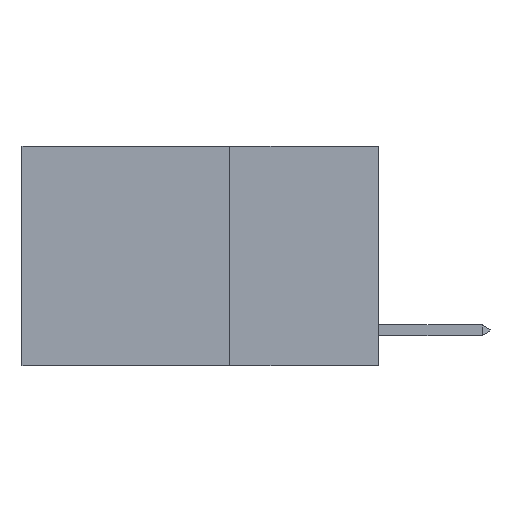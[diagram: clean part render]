
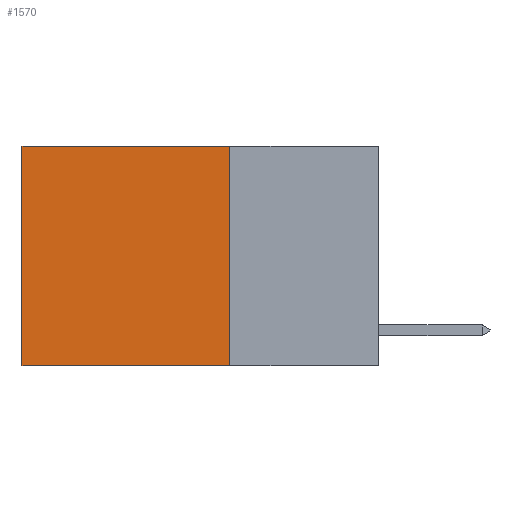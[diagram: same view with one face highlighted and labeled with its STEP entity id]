
A CAD part, left-side view. The second image highlights one B-rep face of the part: STEP entity #1570.
In plain terms, the highlighted planar face has unit normal (-1, 0, 0).
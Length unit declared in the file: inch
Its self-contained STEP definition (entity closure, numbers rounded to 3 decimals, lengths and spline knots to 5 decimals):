
#242 = ORIENTED_EDGE ( 'NONE', *, *, #7234, .T. ) ;
#733 = ORIENTED_EDGE ( 'NONE', *, *, #9183, .F. ) ;
#904 = ORIENTED_EDGE ( 'NONE', *, *, #3686, .T. ) ;
#1250 = VECTOR ( 'NONE', #5497, 39.37008 ) ;
#1519 = VERTEX_POINT ( 'NONE', #7907 ) ;
#1570 = ADVANCED_FACE ( 'NONE', ( #4399 ), #10146, .F. ) ;
#1814 = ORIENTED_EDGE ( 'NONE', *, *, #3489, .F. ) ;
#2199 = CARTESIAN_POINT ( 'NONE',  ( 0.2625, 0.25, 0. ) ) ;
#2363 = CARTESIAN_POINT ( 'NONE',  ( 0.2625, 0.6, 0. ) ) ;
#2517 = DIRECTION ( 'NONE',  ( 0., 1., 0. ) ) ;
#2641 = CARTESIAN_POINT ( 'NONE',  ( 0.2625, 0.6, -0.37 ) ) ;
#2745 = DIRECTION ( 'NONE',  ( 1., 0., 0. ) ) ;
#2793 = AXIS2_PLACEMENT_3D ( 'NONE', #2849, #2745, #8259 ) ;
#2840 = EDGE_LOOP ( 'NONE', ( #904, #733, #1814, #242 ) ) ;
#2849 = CARTESIAN_POINT ( 'NONE',  ( 0.2625, 0.25, 0. ) ) ;
#2933 = CARTESIAN_POINT ( 'NONE',  ( 0.2625, 0.25, -0.37 ) ) ;
#3489 = EDGE_CURVE ( 'NONE', #4246, #3878, #8770, .T. ) ;
#3686 = EDGE_CURVE ( 'NONE', #1519, #10423, #7468, .T. ) ;
#3878 = VERTEX_POINT ( 'NONE', #2933 ) ;
#4150 = DIRECTION ( 'NONE',  ( 0., 1., 0. ) ) ;
#4246 = VERTEX_POINT ( 'NONE', #10127 ) ;
#4399 = FACE_OUTER_BOUND ( 'NONE', #2840, .T. ) ;
#4859 = VECTOR ( 'NONE', #8113, 39.37008 ) ;
#5168 = LINE ( 'NONE', #8264, #7344 ) ;
#5172 = VECTOR ( 'NONE', #4150, 39.37008 ) ;
#5497 = DIRECTION ( 'NONE',  ( 0., 0., -1. ) ) ;
#5906 = LINE ( 'NONE', #9234, #5172 ) ;
#7234 = EDGE_CURVE ( 'NONE', #4246, #1519, #5906, .T. ) ;
#7344 = VECTOR ( 'NONE', #2517, 39.37008 ) ;
#7468 = LINE ( 'NONE', #2363, #4859 ) ;
#7907 = CARTESIAN_POINT ( 'NONE',  ( 0.2625, 0.6, 0. ) ) ;
#8113 = DIRECTION ( 'NONE',  ( 0., 0., -1. ) ) ;
#8259 = DIRECTION ( 'NONE',  ( 0., 0., -1. ) ) ;
#8264 = CARTESIAN_POINT ( 'NONE',  ( 0.2625, 0.25, -0.37 ) ) ;
#8770 = LINE ( 'NONE', #2199, #1250 ) ;
#9183 = EDGE_CURVE ( 'NONE', #3878, #10423, #5168, .T. ) ;
#9234 = CARTESIAN_POINT ( 'NONE',  ( 0.2625, 0.25, 0. ) ) ;
#10127 = CARTESIAN_POINT ( 'NONE',  ( 0.2625, 0.25, 0. ) ) ;
#10146 = PLANE ( 'NONE',  #2793 ) ;
#10423 = VERTEX_POINT ( 'NONE', #2641 ) ;
